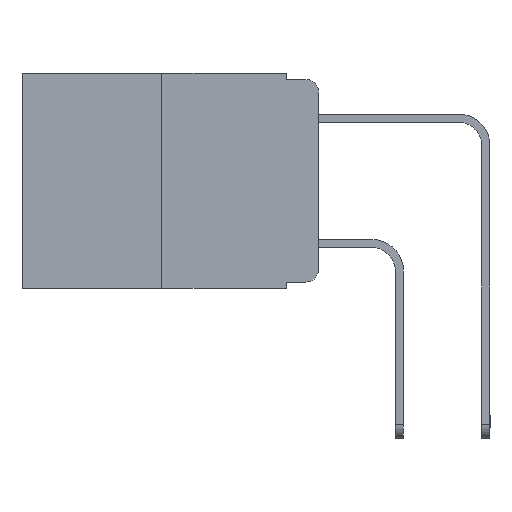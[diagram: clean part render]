
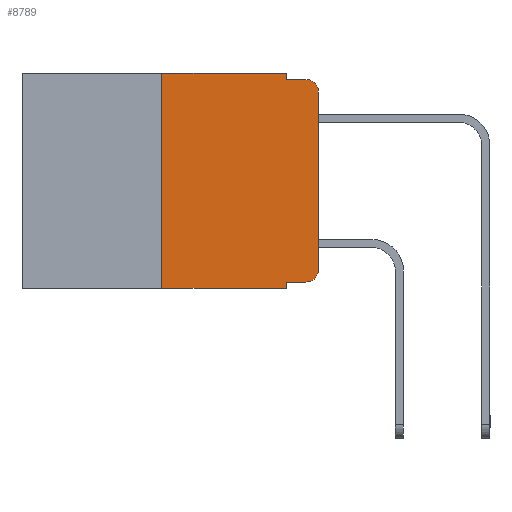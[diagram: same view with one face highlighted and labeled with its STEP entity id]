
A CAD part, left-side view. The second image highlights one B-rep face of the part: STEP entity #8789.
In plain terms, the highlighted planar face has unit normal (-1, 0, 0).
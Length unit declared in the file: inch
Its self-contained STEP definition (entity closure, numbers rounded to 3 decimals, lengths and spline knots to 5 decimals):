
#261 = CARTESIAN_POINT ( 'NONE',  ( 0., 0.473, -0.343 ) ) ;
#575 = ORIENTED_EDGE ( 'NONE', *, *, #7263, .F. ) ;
#703 = CARTESIAN_POINT ( 'NONE',  ( 0., 0.473, 0. ) ) ;
#905 = CIRCLE ( 'NONE', #8105, 0.02 ) ;
#1010 = CARTESIAN_POINT ( 'NONE',  ( 0., 0.051, 0. ) ) ;
#1224 = LINE ( 'NONE', #12135, #12230 ) ;
#1248 = VERTEX_POINT ( 'NONE', #11590 ) ;
#1269 = EDGE_CURVE ( 'NONE', #3125, #5000, #2761, .T. ) ;
#1277 = CARTESIAN_POINT ( 'NONE',  ( 0., 0.02, -0.313 ) ) ;
#1421 = DIRECTION ( 'NONE',  ( 0., -1., 0. ) ) ;
#1808 = CARTESIAN_POINT ( 'NONE',  ( 0., 0.25, -0.343 ) ) ;
#1847 = EDGE_CURVE ( 'NONE', #5279, #8083, #2906, .T. ) ;
#1882 = CARTESIAN_POINT ( 'NONE',  ( 0., 0.25, 0. ) ) ;
#2012 = EDGE_CURVE ( 'NONE', #6752, #3125, #4091, .T. ) ;
#2185 = DIRECTION ( 'NONE',  ( 0., 0., -1. ) ) ;
#2351 = AXIS2_PLACEMENT_3D ( 'NONE', #8163, #10066, #6328 ) ;
#2406 = PLANE ( 'NONE',  #2351 ) ;
#2733 = VERTEX_POINT ( 'NONE', #12700 ) ;
#2761 = LINE ( 'NONE', #9724, #10543 ) ;
#2906 = LINE ( 'NONE', #6827, #8097 ) ;
#3125 = VERTEX_POINT ( 'NONE', #9877 ) ;
#3325 = CARTESIAN_POINT ( 'NONE',  ( 0., 0.02, -0.01 ) ) ;
#3359 = DIRECTION ( 'NONE',  ( 0., 0., -1. ) ) ;
#3807 = LINE ( 'NONE', #703, #5815 ) ;
#4091 = LINE ( 'NONE', #8024, #11819 ) ;
#4105 = LINE ( 'NONE', #5125, #11026 ) ;
#4339 = FACE_OUTER_BOUND ( 'NONE', #8948, .T. ) ;
#4351 = DIRECTION ( 'NONE',  ( -1., 0., 0. ) ) ;
#4641 = DIRECTION ( 'NONE',  ( 0., -1., 0. ) ) ;
#4987 = EDGE_CURVE ( 'NONE', #1248, #5377, #4105, .T. ) ;
#5000 = VERTEX_POINT ( 'NONE', #3325 ) ;
#5125 = CARTESIAN_POINT ( 'NONE',  ( 0., 0., 0. ) ) ;
#5234 = ORIENTED_EDGE ( 'NONE', *, *, #7594, .T. ) ;
#5279 = VERTEX_POINT ( 'NONE', #6605 ) ;
#5377 = VERTEX_POINT ( 'NONE', #9763 ) ;
#5815 = VECTOR ( 'NONE', #4641, 39.37008 ) ;
#6097 = VECTOR ( 'NONE', #2185, 39.37008 ) ;
#6292 = ORIENTED_EDGE ( 'NONE', *, *, #7468, .F. ) ;
#6328 = DIRECTION ( 'NONE',  ( 0., 0., -1. ) ) ;
#6605 = CARTESIAN_POINT ( 'NONE',  ( 0., 0.051, -0.333 ) ) ;
#6647 = VERTEX_POINT ( 'NONE', #1882 ) ;
#6752 = VERTEX_POINT ( 'NONE', #1010 ) ;
#6827 = CARTESIAN_POINT ( 'NONE',  ( 0., 0.051, -0.333 ) ) ;
#7020 = ORIENTED_EDGE ( 'NONE', *, *, #10498, .T. ) ;
#7042 = VERTEX_POINT ( 'NONE', #1808 ) ;
#7121 = ORIENTED_EDGE ( 'NONE', *, *, #12489, .T. ) ;
#7263 = EDGE_CURVE ( 'NONE', #7042, #6647, #1224, .T. ) ;
#7468 = EDGE_CURVE ( 'NONE', #6647, #6752, #3807, .T. ) ;
#7594 = EDGE_CURVE ( 'NONE', #5377, #5000, #905, .T. ) ;
#7801 = CARTESIAN_POINT ( 'NONE',  ( 0., 0.02, -0.333 ) ) ;
#8008 = ORIENTED_EDGE ( 'NONE', *, *, #1847, .T. ) ;
#8024 = CARTESIAN_POINT ( 'NONE',  ( 0., 0.051, 0. ) ) ;
#8083 = VERTEX_POINT ( 'NONE', #7801 ) ;
#8097 = VECTOR ( 'NONE', #10750, 39.37008 ) ;
#8105 = AXIS2_PLACEMENT_3D ( 'NONE', #10877, #4351, #9191 ) ;
#8163 = CARTESIAN_POINT ( 'NONE',  ( 0., 0.473, 0. ) ) ;
#8171 = DIRECTION ( 'NONE',  ( 0., 0., 1. ) ) ;
#8762 = VECTOR ( 'NONE', #1421, 39.37008 ) ;
#8789 = ADVANCED_FACE ( 'NONE', ( #4339 ), #2406, .F. ) ;
#8790 = ORIENTED_EDGE ( 'NONE', *, *, #2012, .F. ) ;
#8948 = EDGE_LOOP ( 'NONE', ( #11050, #5234, #9941, #8790, #6292, #575, #7020, #10803, #8008, #7121 ) ) ;
#9038 = DIRECTION ( 'NONE',  ( 0., 0., 1. ) ) ;
#9191 = DIRECTION ( 'NONE',  ( 0., 0., -1. ) ) ;
#9724 = CARTESIAN_POINT ( 'NONE',  ( 0., 0.051, -0.01 ) ) ;
#9763 = CARTESIAN_POINT ( 'NONE',  ( 0., 0., -0.03 ) ) ;
#9874 = CARTESIAN_POINT ( 'NONE',  ( 0., 0.051, 0. ) ) ;
#9877 = CARTESIAN_POINT ( 'NONE',  ( 0., 0.051, -0.01 ) ) ;
#9941 = ORIENTED_EDGE ( 'NONE', *, *, #1269, .F. ) ;
#10066 = DIRECTION ( 'NONE',  ( 1., 0., 0. ) ) ;
#10258 = LINE ( 'NONE', #261, #8762 ) ;
#10498 = EDGE_CURVE ( 'NONE', #7042, #2733, #10258, .T. ) ;
#10543 = VECTOR ( 'NONE', #12634, 39.37008 ) ;
#10635 = AXIS2_PLACEMENT_3D ( 'NONE', #1277, #12068, #3359 ) ;
#10750 = DIRECTION ( 'NONE',  ( 0., -1., 0. ) ) ;
#10803 = ORIENTED_EDGE ( 'NONE', *, *, #12382, .F. ) ;
#10877 = CARTESIAN_POINT ( 'NONE',  ( 0., 0.02, -0.03 ) ) ;
#11026 = VECTOR ( 'NONE', #8171, 39.37008 ) ;
#11038 = DIRECTION ( 'NONE',  ( 0., 0., -1. ) ) ;
#11050 = ORIENTED_EDGE ( 'NONE', *, *, #4987, .T. ) ;
#11262 = CIRCLE ( 'NONE', #10635, 0.02 ) ;
#11590 = CARTESIAN_POINT ( 'NONE',  ( 0., 0., -0.313 ) ) ;
#11819 = VECTOR ( 'NONE', #11038, 39.37008 ) ;
#12068 = DIRECTION ( 'NONE',  ( -1., 0., 0. ) ) ;
#12135 = CARTESIAN_POINT ( 'NONE',  ( 0., 0.25, 0. ) ) ;
#12230 = VECTOR ( 'NONE', #9038, 39.37008 ) ;
#12382 = EDGE_CURVE ( 'NONE', #5279, #2733, #12738, .T. ) ;
#12489 = EDGE_CURVE ( 'NONE', #8083, #1248, #11262, .T. ) ;
#12634 = DIRECTION ( 'NONE',  ( 0., -1., 0. ) ) ;
#12700 = CARTESIAN_POINT ( 'NONE',  ( 0., 0.051, -0.343 ) ) ;
#12738 = LINE ( 'NONE', #9874, #6097 ) ;
